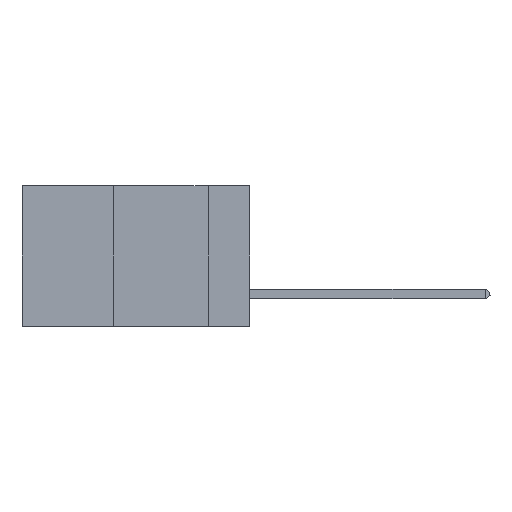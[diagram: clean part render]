
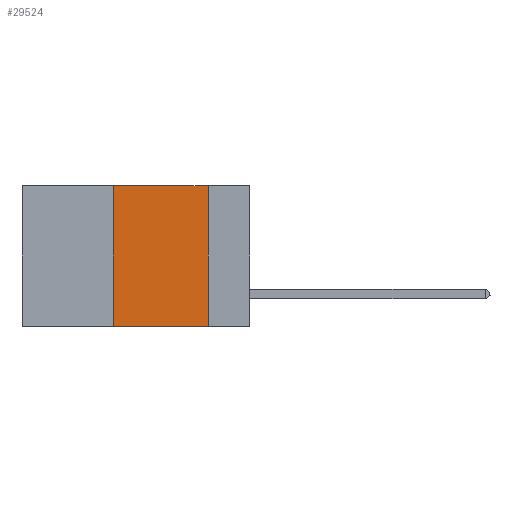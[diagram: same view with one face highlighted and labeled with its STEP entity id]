
A CAD part, left-side view. The second image highlights one B-rep face of the part: STEP entity #29524.
In plain terms, the highlighted planar face has unit normal (-1, 0, 0).
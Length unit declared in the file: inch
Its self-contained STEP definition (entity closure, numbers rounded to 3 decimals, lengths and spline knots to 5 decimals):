
#275 = DIRECTION ( 'NONE',  ( 0., 0., -1. ) ) ;
#7403 = DIRECTION ( 'NONE',  ( 0., 0., 1. ) ) ;
#8977 = CARTESIAN_POINT ( 'NONE',  ( 0., 0.6, -0.37 ) ) ;
#10337 = DIRECTION ( 'NONE',  ( 1., 0., 0. ) ) ;
#11075 = CARTESIAN_POINT ( 'NONE',  ( 0., 0.6, 0. ) ) ;
#12660 = VECTOR ( 'NONE', #275, 39.37008 ) ;
#14222 = PLANE ( 'NONE',  #38246 ) ;
#14224 = VECTOR ( 'NONE', #33865, 39.37008 ) ;
#14499 = EDGE_CURVE ( 'NONE', #23351, #23541, #19071, .T. ) ;
#19071 = LINE ( 'NONE', #28576, #40192 ) ;
#21667 = LINE ( 'NONE', #11075, #32258 ) ;
#21900 = ORIENTED_EDGE ( 'NONE', *, *, #14499, .F. ) ;
#22009 = EDGE_CURVE ( 'NONE', #23351, #40942, #22546, .T. ) ;
#22128 = CARTESIAN_POINT ( 'NONE',  ( 0., 0.11, 0. ) ) ;
#22546 = LINE ( 'NONE', #8977, #14224 ) ;
#22857 = CARTESIAN_POINT ( 'NONE',  ( 0., 0.36, 0. ) ) ;
#23351 = VERTEX_POINT ( 'NONE', #25219 ) ;
#23429 = EDGE_CURVE ( 'NONE', #23541, #34031, #21667, .T. ) ;
#23541 = VERTEX_POINT ( 'NONE', #22857 ) ;
#24632 = CARTESIAN_POINT ( 'NONE',  ( 0., 0.6, 0. ) ) ;
#25219 = CARTESIAN_POINT ( 'NONE',  ( 0., 0.36, -0.37 ) ) ;
#25615 = ORIENTED_EDGE ( 'NONE', *, *, #22009, .T. ) ;
#28576 = CARTESIAN_POINT ( 'NONE',  ( 0., 0.36, 0. ) ) ;
#29524 = ADVANCED_FACE ( 'NONE', ( #34624 ), #14222, .F. ) ;
#31962 = DIRECTION ( 'NONE',  ( 0., 0., -1. ) ) ;
#32258 = VECTOR ( 'NONE', #32685, 39.37008 ) ;
#32685 = DIRECTION ( 'NONE',  ( 0., -1., 0. ) ) ;
#32704 = ORIENTED_EDGE ( 'NONE', *, *, #23429, .F. ) ;
#32746 = EDGE_CURVE ( 'NONE', #34031, #40942, #43268, .T. ) ;
#33226 = CARTESIAN_POINT ( 'NONE',  ( 0., 0.11, -0.37 ) ) ;
#33865 = DIRECTION ( 'NONE',  ( 0., -1., 0. ) ) ;
#34031 = VERTEX_POINT ( 'NONE', #22128 ) ;
#34624 = FACE_OUTER_BOUND ( 'NONE', #40571, .T. ) ;
#34784 = ORIENTED_EDGE ( 'NONE', *, *, #32746, .F. ) ;
#35944 = CARTESIAN_POINT ( 'NONE',  ( 0., 0.11, 0. ) ) ;
#38246 = AXIS2_PLACEMENT_3D ( 'NONE', #24632, #10337, #31962 ) ;
#40192 = VECTOR ( 'NONE', #7403, 39.37008 ) ;
#40571 = EDGE_LOOP ( 'NONE', ( #34784, #32704, #21900, #25615 ) ) ;
#40942 = VERTEX_POINT ( 'NONE', #33226 ) ;
#43268 = LINE ( 'NONE', #35944, #12660 ) ;
